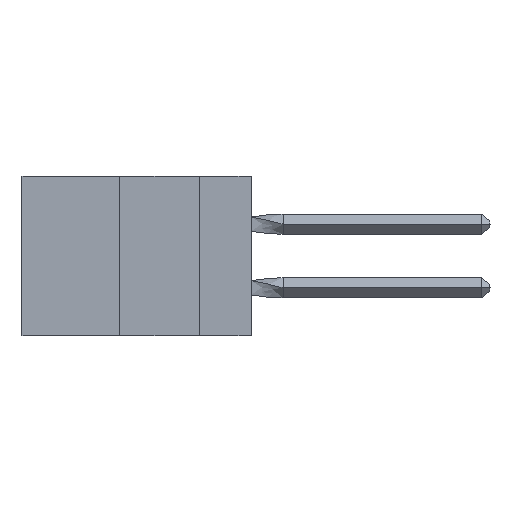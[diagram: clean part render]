
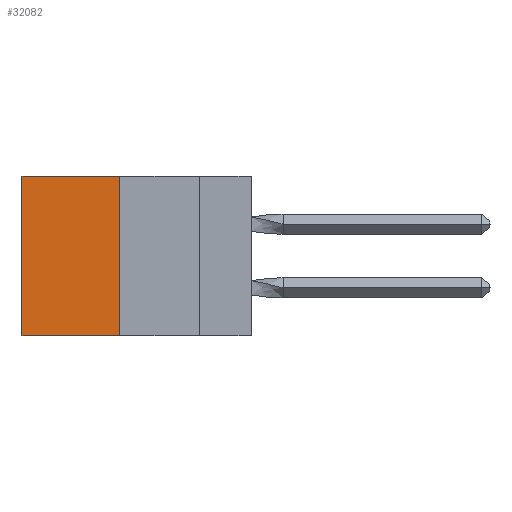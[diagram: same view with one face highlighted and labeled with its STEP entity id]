
A CAD part, left-side view. The second image highlights one B-rep face of the part: STEP entity #32082.
In plain terms, the highlighted planar face has unit normal (-1, 0, 0).
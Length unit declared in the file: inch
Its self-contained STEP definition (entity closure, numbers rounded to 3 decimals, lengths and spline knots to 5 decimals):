
#405 = CARTESIAN_POINT ( 'NONE',  ( 0.305, 0.72, 0. ) ) ;
#580 = CARTESIAN_POINT ( 'NONE',  ( 0.305, 0.413, -0.5 ) ) ;
#1774 = ORIENTED_EDGE ( 'NONE', *, *, #27592, .F. ) ;
#3265 = ORIENTED_EDGE ( 'NONE', *, *, #5110, .F. ) ;
#4381 = AXIS2_PLACEMENT_3D ( 'NONE', #17139, #4552, #7286 ) ;
#4552 = DIRECTION ( 'NONE',  ( 1., 0., 0. ) ) ;
#5110 = EDGE_CURVE ( 'NONE', #7437, #39023, #9256, .T. ) ;
#7286 = DIRECTION ( 'NONE',  ( 0., 0., -1. ) ) ;
#7336 = LINE ( 'NONE', #580, #41006 ) ;
#7437 = VERTEX_POINT ( 'NONE', #10547 ) ;
#8551 = VECTOR ( 'NONE', #34355, 39.37008 ) ;
#9256 = LINE ( 'NONE', #23824, #33782 ) ;
#10547 = CARTESIAN_POINT ( 'NONE',  ( 0.305, 0.413, 0. ) ) ;
#10956 = PLANE ( 'NONE',  #4381 ) ;
#14130 = EDGE_CURVE ( 'NONE', #7437, #31935, #17811, .T. ) ;
#16251 = CARTESIAN_POINT ( 'NONE',  ( 0.305, 0.413, -0.5 ) ) ;
#17139 = CARTESIAN_POINT ( 'NONE',  ( 0.305, 0.413, -0.5 ) ) ;
#17811 = LINE ( 'NONE', #40922, #8551 ) ;
#18621 = LINE ( 'NONE', #41367, #41556 ) ;
#19441 = ORIENTED_EDGE ( 'NONE', *, *, #23940, .T. ) ;
#20342 = DIRECTION ( 'NONE',  ( 0., 1., 0. ) ) ;
#23824 = CARTESIAN_POINT ( 'NONE',  ( 0.305, 0.413, -0.5 ) ) ;
#23940 = EDGE_CURVE ( 'NONE', #31935, #24958, #18621, .T. ) ;
#24958 = VERTEX_POINT ( 'NONE', #35356 ) ;
#27117 = DIRECTION ( 'NONE',  ( 0., 0., -1. ) ) ;
#27592 = EDGE_CURVE ( 'NONE', #39023, #24958, #7336, .T. ) ;
#27803 = ORIENTED_EDGE ( 'NONE', *, *, #14130, .T. ) ;
#29007 = FACE_OUTER_BOUND ( 'NONE', #33720, .T. ) ;
#31484 = DIRECTION ( 'NONE',  ( 0., 0., -1. ) ) ;
#31935 = VERTEX_POINT ( 'NONE', #405 ) ;
#32082 = ADVANCED_FACE ( 'NONE', ( #29007 ), #10956, .F. ) ;
#33720 = EDGE_LOOP ( 'NONE', ( #19441, #1774, #3265, #27803 ) ) ;
#33782 = VECTOR ( 'NONE', #27117, 39.37008 ) ;
#34355 = DIRECTION ( 'NONE',  ( 0., 1., 0. ) ) ;
#35356 = CARTESIAN_POINT ( 'NONE',  ( 0.305, 0.72, -0.5 ) ) ;
#39023 = VERTEX_POINT ( 'NONE', #16251 ) ;
#40922 = CARTESIAN_POINT ( 'NONE',  ( 0.305, 0.413, 0. ) ) ;
#41006 = VECTOR ( 'NONE', #20342, 39.37008 ) ;
#41367 = CARTESIAN_POINT ( 'NONE',  ( 0.305, 0.72, -0.5 ) ) ;
#41556 = VECTOR ( 'NONE', #31484, 39.37008 ) ;
